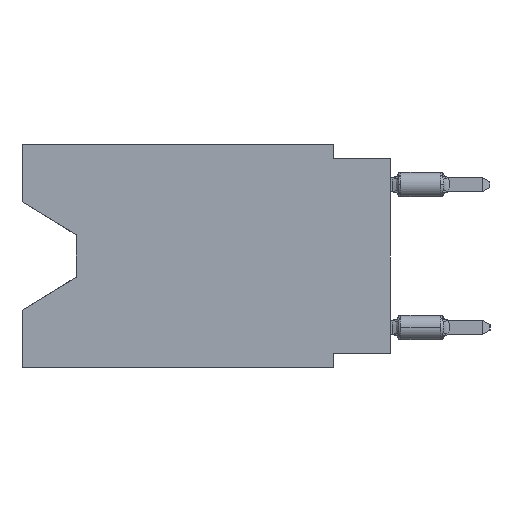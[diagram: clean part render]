
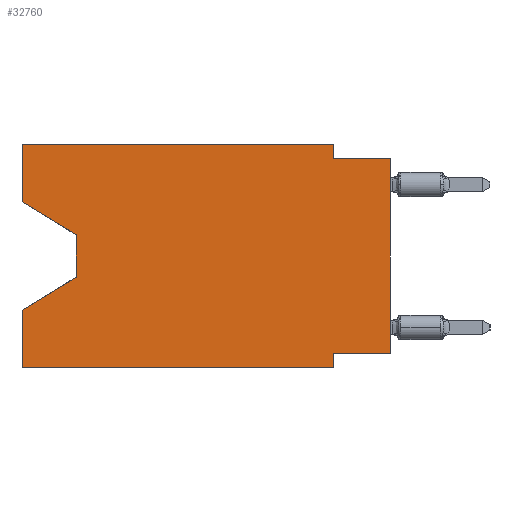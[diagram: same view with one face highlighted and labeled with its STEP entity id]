
A CAD part, left-side view. The second image highlights one B-rep face of the part: STEP entity #32760.
In plain terms, the highlighted planar face has unit normal (-1, 0, 0).
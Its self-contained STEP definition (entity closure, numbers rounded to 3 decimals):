
#23 = VECTOR ( 'NONE', #11034, 1000. ) ;
#312 = LINE ( 'NONE', #5995, #5488 ) ;
#331 = LINE ( 'NONE', #3254, #23 ) ;
#617 = LINE ( 'NONE', #21622, #19953 ) ;
#708 = ORIENTED_EDGE ( 'NONE', *, *, #32317, .T. ) ;
#954 = DIRECTION ( 'NONE',  ( 0., 1., 0. ) ) ;
#1335 = CARTESIAN_POINT ( 'NONE',  ( 0., 0., -0.635 ) ) ;
#1886 = LINE ( 'NONE', #14800, #17113 ) ;
#2079 = LINE ( 'NONE', #6581, #23308 ) ;
#3196 = CARTESIAN_POINT ( 'NONE',  ( 0., 0., -9.271 ) ) ;
#3254 = CARTESIAN_POINT ( 'NONE',  ( 0., 13.97, -4.013 ) ) ;
#3368 = LINE ( 'NONE', #26934, #32440 ) ;
#3376 = CARTESIAN_POINT ( 'NONE',  ( 0., 16.383, -7.36 ) ) ;
#3456 = CARTESIAN_POINT ( 'NONE',  ( 0., 16.383, -2.546 ) ) ;
#3689 = EDGE_CURVE ( 'NONE', #24950, #25148, #29911, .T. ) ;
#4641 = VECTOR ( 'NONE', #6206, 1000. ) ;
#4859 = VERTEX_POINT ( 'NONE', #31626 ) ;
#5474 = ORIENTED_EDGE ( 'NONE', *, *, #30226, .T. ) ;
#5488 = VECTOR ( 'NONE', #11356, 1000. ) ;
#5953 = CARTESIAN_POINT ( 'NONE',  ( 0., 13.97, -5.893 ) ) ;
#5995 = CARTESIAN_POINT ( 'NONE',  ( 0., 0., 0. ) ) ;
#6206 = DIRECTION ( 'NONE',  ( 0., -1., 0. ) ) ;
#6209 = DIRECTION ( 'NONE',  ( 0., -1., 0. ) ) ;
#6442 = VERTEX_POINT ( 'NONE', #32683 ) ;
#6524 = EDGE_CURVE ( 'NONE', #6442, #21810, #10175, .T. ) ;
#6581 = CARTESIAN_POINT ( 'NONE',  ( 0., 2.54, 0. ) ) ;
#7237 = CARTESIAN_POINT ( 'NONE',  ( 0., 2.54, -9.906 ) ) ;
#7255 = VERTEX_POINT ( 'NONE', #5953 ) ;
#8339 = FACE_OUTER_BOUND ( 'NONE', #15111, .T. ) ;
#8509 = CARTESIAN_POINT ( 'NONE',  ( 0., 16.383, 0. ) ) ;
#8513 = VERTEX_POINT ( 'NONE', #23941 ) ;
#8622 = CARTESIAN_POINT ( 'NONE',  ( 0., 16.383, -9.906 ) ) ;
#9297 = LINE ( 'NONE', #8622, #31901 ) ;
#9766 = EDGE_CURVE ( 'NONE', #29343, #24950, #2079, .T. ) ;
#9926 = CARTESIAN_POINT ( 'NONE',  ( 0., 13.97, -4.013 ) ) ;
#10175 = LINE ( 'NONE', #7237, #23394 ) ;
#11034 = DIRECTION ( 'NONE',  ( 0., 0., -1. ) ) ;
#11196 = VERTEX_POINT ( 'NONE', #27534 ) ;
#11264 = DIRECTION ( 'NONE',  ( 0., -0.855, -0.519 ) ) ;
#11356 = DIRECTION ( 'NONE',  ( 0., 0., 1. ) ) ;
#12058 = DIRECTION ( 'NONE',  ( 0., 0., 1. ) ) ;
#13840 = EDGE_CURVE ( 'NONE', #31592, #21217, #31535, .T. ) ;
#13964 = LINE ( 'NONE', #16538, #4641 ) ;
#14266 = DIRECTION ( 'NONE',  ( 0., -1., 0. ) ) ;
#14516 = DIRECTION ( 'NONE',  ( 0., 0., -1. ) ) ;
#14660 = ORIENTED_EDGE ( 'NONE', *, *, #19544, .T. ) ;
#14678 = EDGE_CURVE ( 'NONE', #31592, #11196, #3368, .T. ) ;
#14708 = ORIENTED_EDGE ( 'NONE', *, *, #3689, .F. ) ;
#14800 = CARTESIAN_POINT ( 'NONE',  ( 0., 16.383, 0. ) ) ;
#14883 = ORIENTED_EDGE ( 'NONE', *, *, #16833, .T. ) ;
#15111 = EDGE_LOOP ( 'NONE', ( #27139, #14660, #708, #24529, #5474, #22991, #31517, #14883, #14708, #25927, #22268, #21354 ) ) ;
#16264 = PLANE ( 'NONE',  #29814 ) ;
#16538 = CARTESIAN_POINT ( 'NONE',  ( 0., 16.383, 0. ) ) ;
#16810 = LINE ( 'NONE', #3196, #21051 ) ;
#16833 = EDGE_CURVE ( 'NONE', #4859, #25148, #312, .T. ) ;
#17113 = VECTOR ( 'NONE', #12058, 1000. ) ;
#17976 = CARTESIAN_POINT ( 'NONE',  ( 0., 2.54, -9.906 ) ) ;
#18417 = CARTESIAN_POINT ( 'NONE',  ( 0., 2.54, -0.635 ) ) ;
#18842 = DIRECTION ( 'NONE',  ( 1., 0., 0. ) ) ;
#18997 = CARTESIAN_POINT ( 'NONE',  ( 0., 16.383, -2.546 ) ) ;
#19006 = DIRECTION ( 'NONE',  ( 0., 0., -1. ) ) ;
#19544 = EDGE_CURVE ( 'NONE', #21217, #7255, #331, .T. ) ;
#19953 = VECTOR ( 'NONE', #24372, 1000. ) ;
#20480 = DIRECTION ( 'NONE',  ( 0., 0., -1. ) ) ;
#21051 = VECTOR ( 'NONE', #954, 1000. ) ;
#21217 = VERTEX_POINT ( 'NONE', #9926 ) ;
#21354 = ORIENTED_EDGE ( 'NONE', *, *, #14678, .F. ) ;
#21622 = CARTESIAN_POINT ( 'NONE',  ( 0., 13.97, -5.893 ) ) ;
#21810 = VERTEX_POINT ( 'NONE', #17976 ) ;
#22268 = ORIENTED_EDGE ( 'NONE', *, *, #22290, .F. ) ;
#22290 = EDGE_CURVE ( 'NONE', #11196, #29343, #13964, .T. ) ;
#22991 = ORIENTED_EDGE ( 'NONE', *, *, #6524, .F. ) ;
#23308 = VECTOR ( 'NONE', #14516, 1000. ) ;
#23394 = VECTOR ( 'NONE', #20480, 1000. ) ;
#23941 = CARTESIAN_POINT ( 'NONE',  ( 0., 16.383, -9.906 ) ) ;
#24017 = DIRECTION ( 'NONE',  ( 0., 0., 1. ) ) ;
#24372 = DIRECTION ( 'NONE',  ( 0., 0.855, -0.519 ) ) ;
#24529 = ORIENTED_EDGE ( 'NONE', *, *, #30433, .F. ) ;
#24950 = VERTEX_POINT ( 'NONE', #18417 ) ;
#25148 = VERTEX_POINT ( 'NONE', #26808 ) ;
#25927 = ORIENTED_EDGE ( 'NONE', *, *, #9766, .F. ) ;
#26808 = CARTESIAN_POINT ( 'NONE',  ( 0., 0., -0.635 ) ) ;
#26934 = CARTESIAN_POINT ( 'NONE',  ( 0., 16.383, 0. ) ) ;
#27139 = ORIENTED_EDGE ( 'NONE', *, *, #13840, .T. ) ;
#27377 = VERTEX_POINT ( 'NONE', #3376 ) ;
#27534 = CARTESIAN_POINT ( 'NONE',  ( 0., 16.383, 0. ) ) ;
#29343 = VERTEX_POINT ( 'NONE', #32238 ) ;
#29814 = AXIS2_PLACEMENT_3D ( 'NONE', #8509, #18842, #19006 ) ;
#29911 = LINE ( 'NONE', #1335, #33878 ) ;
#30183 = VECTOR ( 'NONE', #11264, 1000. ) ;
#30226 = EDGE_CURVE ( 'NONE', #8513, #21810, #9297, .T. ) ;
#30433 = EDGE_CURVE ( 'NONE', #8513, #27377, #1886, .T. ) ;
#31517 = ORIENTED_EDGE ( 'NONE', *, *, #32335, .F. ) ;
#31535 = LINE ( 'NONE', #18997, #30183 ) ;
#31592 = VERTEX_POINT ( 'NONE', #3456 ) ;
#31626 = CARTESIAN_POINT ( 'NONE',  ( 0., 0., -9.271 ) ) ;
#31901 = VECTOR ( 'NONE', #6209, 1000. ) ;
#32238 = CARTESIAN_POINT ( 'NONE',  ( 0., 2.54, 0. ) ) ;
#32317 = EDGE_CURVE ( 'NONE', #7255, #27377, #617, .T. ) ;
#32335 = EDGE_CURVE ( 'NONE', #4859, #6442, #16810, .T. ) ;
#32440 = VECTOR ( 'NONE', #24017, 1000. ) ;
#32683 = CARTESIAN_POINT ( 'NONE',  ( 0., 2.54, -9.271 ) ) ;
#32760 = ADVANCED_FACE ( 'NONE', ( #8339 ), #16264, .F. ) ;
#33878 = VECTOR ( 'NONE', #14266, 1000. ) ;
